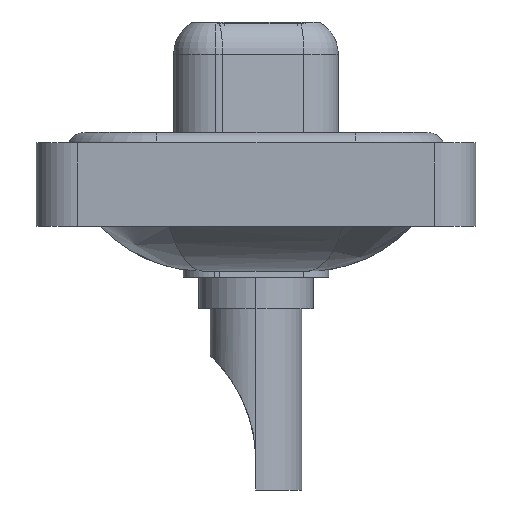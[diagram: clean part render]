
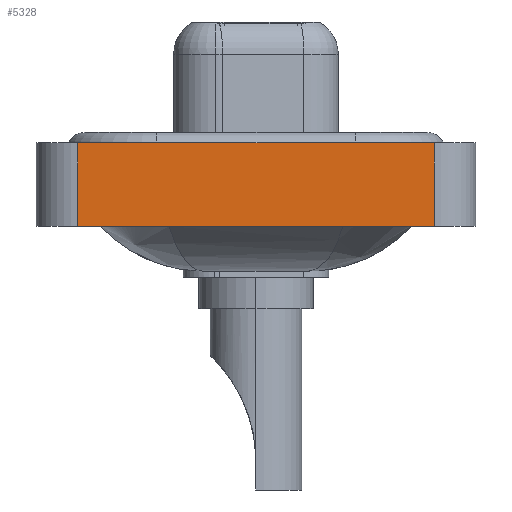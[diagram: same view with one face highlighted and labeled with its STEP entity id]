
A CAD part, left-side view. The second image highlights one B-rep face of the part: STEP entity #5328.
In plain terms, the highlighted planar face has unit normal (-1, 0, 0).
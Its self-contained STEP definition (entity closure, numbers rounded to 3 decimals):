
#876 = CARTESIAN_POINT ( 'NONE',  ( -7.3, 8.55, -3.6 ) ) ;
#884 = ORIENTED_EDGE ( 'NONE', *, *, #15294, .T. ) ;
#1335 = VECTOR ( 'NONE', #12722, 1000. ) ;
#3679 = VERTEX_POINT ( 'NONE', #11238 ) ;
#3703 = ORIENTED_EDGE ( 'NONE', *, *, #8459, .F. ) ;
#3954 = DIRECTION ( 'NONE',  ( -1., 0., 0. ) ) ;
#4108 = CARTESIAN_POINT ( 'NONE',  ( -7.3, 8.55, 0.4 ) ) ;
#5328 = ADVANCED_FACE ( 'NONE', ( #11130 ), #6315, .T. ) ;
#5680 = LINE ( 'NONE', #876, #11586 ) ;
#6315 = PLANE ( 'NONE',  #12256 ) ;
#6320 = ORIENTED_EDGE ( 'NONE', *, *, #6546, .T. ) ;
#6546 = EDGE_CURVE ( 'NONE', #3679, #6988, #6733, .T. ) ;
#6643 = CARTESIAN_POINT ( 'NONE',  ( -7.3, -8.55, -3.6 ) ) ;
#6733 = LINE ( 'NONE', #7714, #1335 ) ;
#6988 = VERTEX_POINT ( 'NONE', #12698 ) ;
#7602 = CARTESIAN_POINT ( 'NONE',  ( -7.3, -8.55, -3.6 ) ) ;
#7714 = CARTESIAN_POINT ( 'NONE',  ( -7.3, -8.55, -3.6 ) ) ;
#8274 = EDGE_CURVE ( 'NONE', #9156, #6988, #11798, .T. ) ;
#8459 = EDGE_CURVE ( 'NONE', #11037, #9156, #5680, .T. ) ;
#8828 = VECTOR ( 'NONE', #8995, 1000. ) ;
#8995 = DIRECTION ( 'NONE',  ( 0., -1., 0. ) ) ;
#9156 = VERTEX_POINT ( 'NONE', #4108 ) ;
#9333 = DIRECTION ( 'NONE',  ( 0., -1., 0. ) ) ;
#9661 = DIRECTION ( 'NONE',  ( 0., 0., 1. ) ) ;
#9833 = ORIENTED_EDGE ( 'NONE', *, *, #8274, .F. ) ;
#11037 = VERTEX_POINT ( 'NONE', #14605 ) ;
#11130 = FACE_OUTER_BOUND ( 'NONE', #14860, .T. ) ;
#11238 = CARTESIAN_POINT ( 'NONE',  ( -7.3, -8.55, -3.6 ) ) ;
#11586 = VECTOR ( 'NONE', #9661, 1000. ) ;
#11695 = LINE ( 'NONE', #6643, #8828 ) ;
#11798 = LINE ( 'NONE', #15538, #14686 ) ;
#12256 = AXIS2_PLACEMENT_3D ( 'NONE', #7602, #3954, #13908 ) ;
#12698 = CARTESIAN_POINT ( 'NONE',  ( -7.3, -8.55, 0.4 ) ) ;
#12722 = DIRECTION ( 'NONE',  ( 0., 0., 1. ) ) ;
#13908 = DIRECTION ( 'NONE',  ( 0., 0., 1. ) ) ;
#14605 = CARTESIAN_POINT ( 'NONE',  ( -7.3, 8.55, -3.6 ) ) ;
#14686 = VECTOR ( 'NONE', #9333, 1000. ) ;
#14860 = EDGE_LOOP ( 'NONE', ( #6320, #9833, #3703, #884 ) ) ;
#15294 = EDGE_CURVE ( 'NONE', #11037, #3679, #11695, .T. ) ;
#15538 = CARTESIAN_POINT ( 'NONE',  ( -7.3, -8.55, 0.4 ) ) ;
